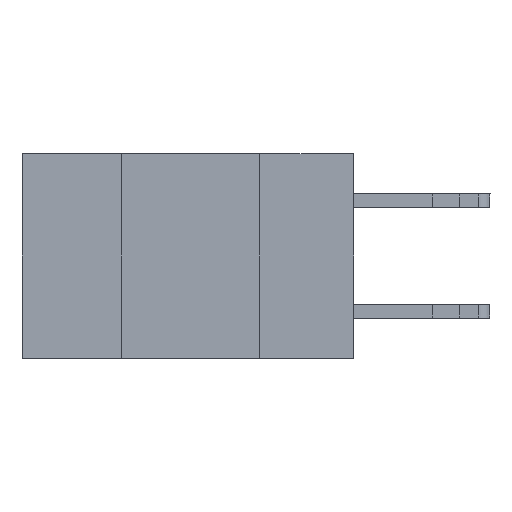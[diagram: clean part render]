
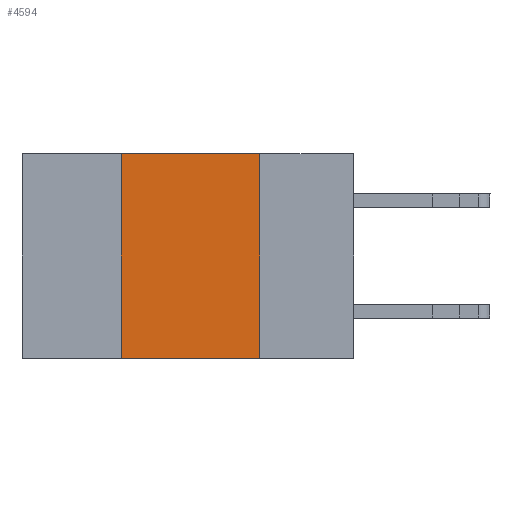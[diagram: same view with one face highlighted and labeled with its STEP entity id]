
A CAD part, left-side view. The second image highlights one B-rep face of the part: STEP entity #4594.
In plain terms, the highlighted planar face has unit normal (-1, 0, 0).
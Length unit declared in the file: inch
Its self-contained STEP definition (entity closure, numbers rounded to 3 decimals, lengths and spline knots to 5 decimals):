
#781 = VECTOR ( 'NONE', #25944, 39.37008 ) ;
#1597 = CARTESIAN_POINT ( 'NONE',  ( 0., 0.42, 0. ) ) ;
#3496 = CARTESIAN_POINT ( 'NONE',  ( 0., 0.6, 0. ) ) ;
#4012 = VERTEX_POINT ( 'NONE', #8414 ) ;
#4594 = ADVANCED_FACE ( 'NONE', ( #16168 ), #27919, .F. ) ;
#5687 = VERTEX_POINT ( 'NONE', #23325 ) ;
#5778 = EDGE_CURVE ( 'NONE', #32502, #5687, #23784, .T. ) ;
#8341 = VECTOR ( 'NONE', #23687, 39.37008 ) ;
#8414 = CARTESIAN_POINT ( 'NONE',  ( 0., 0.17, -0.37 ) ) ;
#8733 = ORIENTED_EDGE ( 'NONE', *, *, #16511, .T. ) ;
#12404 = VECTOR ( 'NONE', #34720, 39.37008 ) ;
#12679 = LINE ( 'NONE', #18549, #781 ) ;
#12732 = AXIS2_PLACEMENT_3D ( 'NONE', #24712, #24833, #22033 ) ;
#16168 = FACE_OUTER_BOUND ( 'NONE', #23204, .T. ) ;
#16511 = EDGE_CURVE ( 'NONE', #26848, #4012, #12679, .T. ) ;
#16905 = EDGE_CURVE ( 'NONE', #26848, #32502, #34395, .T. ) ;
#18549 = CARTESIAN_POINT ( 'NONE',  ( 0., 0.6, -0.37 ) ) ;
#19639 = ORIENTED_EDGE ( 'NONE', *, *, #16905, .F. ) ;
#20228 = EDGE_CURVE ( 'NONE', #5687, #4012, #36414, .T. ) ;
#21552 = DIRECTION ( 'NONE',  ( 0., 0., 1. ) ) ;
#22033 = DIRECTION ( 'NONE',  ( 0., 0., -1. ) ) ;
#22484 = CARTESIAN_POINT ( 'NONE',  ( 0., 0.42, -0.37 ) ) ;
#23204 = EDGE_LOOP ( 'NONE', ( #29381, #33294, #19639, #8733 ) ) ;
#23325 = CARTESIAN_POINT ( 'NONE',  ( 0., 0.17, 0. ) ) ;
#23687 = DIRECTION ( 'NONE',  ( 0., -1., 0. ) ) ;
#23784 = LINE ( 'NONE', #3496, #8341 ) ;
#24712 = CARTESIAN_POINT ( 'NONE',  ( 0., 0.6, 0. ) ) ;
#24833 = DIRECTION ( 'NONE',  ( 1., 0., 0. ) ) ;
#25944 = DIRECTION ( 'NONE',  ( 0., -1., 0. ) ) ;
#26848 = VERTEX_POINT ( 'NONE', #22484 ) ;
#27919 = PLANE ( 'NONE',  #12732 ) ;
#28798 = CARTESIAN_POINT ( 'NONE',  ( 0., 0.42, 0. ) ) ;
#29381 = ORIENTED_EDGE ( 'NONE', *, *, #20228, .F. ) ;
#32502 = VERTEX_POINT ( 'NONE', #28798 ) ;
#33294 = ORIENTED_EDGE ( 'NONE', *, *, #5778, .F. ) ;
#34395 = LINE ( 'NONE', #1597, #35735 ) ;
#34720 = DIRECTION ( 'NONE',  ( 0., 0., -1. ) ) ;
#35735 = VECTOR ( 'NONE', #21552, 39.37008 ) ;
#36414 = LINE ( 'NONE', #37246, #12404 ) ;
#37246 = CARTESIAN_POINT ( 'NONE',  ( 0., 0.17, 0. ) ) ;
